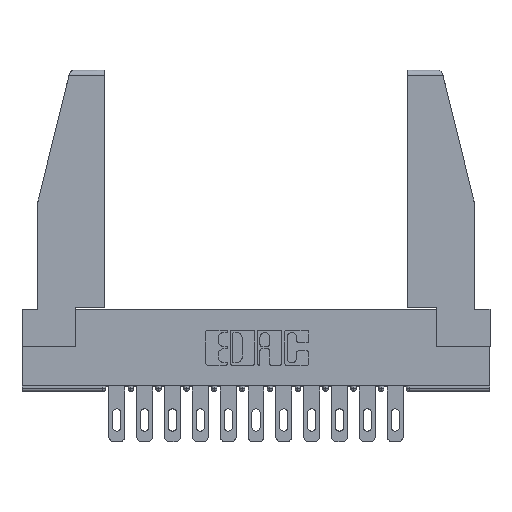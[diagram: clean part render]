
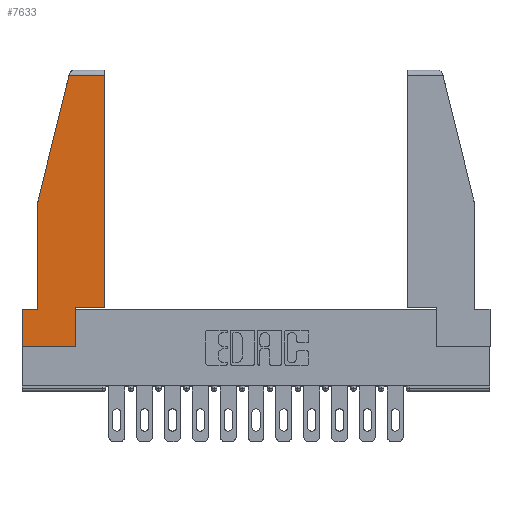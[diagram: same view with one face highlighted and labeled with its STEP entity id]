
A CAD part, top view. The second image highlights one B-rep face of the part: STEP entity #7633.
In plain terms, the highlighted planar face has unit normal (0, 0, 1).
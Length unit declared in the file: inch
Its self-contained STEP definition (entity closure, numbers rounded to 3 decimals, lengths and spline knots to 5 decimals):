
#5 = CARTESIAN_POINT ( 'NONE',  ( 0.086, 0.8, 0. ) ) ;
#120 = CARTESIAN_POINT ( 'NONE',  ( 0., 0., 0. ) ) ;
#125 = VECTOR ( 'NONE', #3399, 39.37008 ) ;
#659 = VERTEX_POINT ( 'NONE', #16445 ) ;
#862 = DIRECTION ( 'NONE',  ( -1., 0., 0. ) ) ;
#889 = ORIENTED_EDGE ( 'NONE', *, *, #14998, .T. ) ;
#1117 = LINE ( 'NONE', #10937, #11453 ) ;
#1218 = CARTESIAN_POINT ( 'NONE',  ( 0., 0.21, 0. ) ) ;
#1313 = VECTOR ( 'NONE', #11374, 39.37008 ) ;
#1883 = EDGE_CURVE ( 'NONE', #5076, #17336, #9200, .T. ) ;
#2120 = LINE ( 'NONE', #8491, #6727 ) ;
#2678 = LINE ( 'NONE', #7862, #3133 ) ;
#2853 = LINE ( 'NONE', #5, #1313 ) ;
#2906 = DIRECTION ( 'NONE',  ( 1., 0., 0. ) ) ;
#2935 = ORIENTED_EDGE ( 'NONE', *, *, #14769, .T. ) ;
#2953 = ORIENTED_EDGE ( 'NONE', *, *, #5495, .T. ) ;
#3133 = VECTOR ( 'NONE', #862, 39.37008 ) ;
#3399 = DIRECTION ( 'NONE',  ( -0.239, -0.971, 0. ) ) ;
#4115 = VERTEX_POINT ( 'NONE', #8168 ) ;
#4915 = DIRECTION ( 'NONE',  ( 0., 1., 0. ) ) ;
#5076 = VERTEX_POINT ( 'NONE', #9344 ) ;
#5495 = EDGE_CURVE ( 'NONE', #17336, #659, #12413, .T. ) ;
#5651 = EDGE_CURVE ( 'NONE', #8223, #5076, #15651, .T. ) ;
#5708 = PLANE ( 'NONE',  #13709 ) ;
#5934 = CARTESIAN_POINT ( 'NONE',  ( 0.461, 0.223, 0. ) ) ;
#6173 = VERTEX_POINT ( 'NONE', #17697 ) ;
#6325 = CARTESIAN_POINT ( 'NONE',  ( 0.297, 0., 0. ) ) ;
#6475 = EDGE_LOOP ( 'NONE', ( #2953, #10082, #889, #10872, #17646, #7102, #2935, #10143, #6641 ) ) ;
#6641 = ORIENTED_EDGE ( 'NONE', *, *, #1883, .T. ) ;
#6727 = VECTOR ( 'NONE', #2906, 39.37008 ) ;
#7102 = ORIENTED_EDGE ( 'NONE', *, *, #12108, .T. ) ;
#7633 = ADVANCED_FACE ( 'NONE', ( #17396 ), #5708, .T. ) ;
#7862 = CARTESIAN_POINT ( 'NONE',  ( 0., 1.52, 0. ) ) ;
#8168 = CARTESIAN_POINT ( 'NONE',  ( 0., 0., 0. ) ) ;
#8223 = VERTEX_POINT ( 'NONE', #6325 ) ;
#8384 = DIRECTION ( 'NONE',  ( 1., 0., 0. ) ) ;
#8491 = CARTESIAN_POINT ( 'NONE',  ( 0., 0., 0. ) ) ;
#8547 = CARTESIAN_POINT ( 'NONE',  ( 0.086, 0.8, 0. ) ) ;
#8592 = DIRECTION ( 'NONE',  ( 0., 0., 1. ) ) ;
#8653 = DIRECTION ( 'NONE',  ( 1., 0., 0. ) ) ;
#9200 = LINE ( 'NONE', #16771, #12053 ) ;
#9232 = VERTEX_POINT ( 'NONE', #18126 ) ;
#9284 = VERTEX_POINT ( 'NONE', #9942 ) ;
#9344 = CARTESIAN_POINT ( 'NONE',  ( 0.297, 0.223, 0. ) ) ;
#9459 = DIRECTION ( 'NONE',  ( 0., -1., 0. ) ) ;
#9942 = CARTESIAN_POINT ( 'NONE',  ( 0.2636, 1.52, 0. ) ) ;
#10082 = ORIENTED_EDGE ( 'NONE', *, *, #17520, .T. ) ;
#10143 = ORIENTED_EDGE ( 'NONE', *, *, #5651, .T. ) ;
#10469 = LINE ( 'NONE', #11800, #125 ) ;
#10872 = ORIENTED_EDGE ( 'NONE', *, *, #12628, .T. ) ;
#10879 = DIRECTION ( 'NONE',  ( -1., 0., 0. ) ) ;
#10937 = CARTESIAN_POINT ( 'NONE',  ( 0., 0.21, 0. ) ) ;
#11321 = VECTOR ( 'NONE', #4915, 39.37008 ) ;
#11374 = DIRECTION ( 'NONE',  ( 0., -1., 0. ) ) ;
#11453 = VECTOR ( 'NONE', #9459, 39.37008 ) ;
#11800 = CARTESIAN_POINT ( 'NONE',  ( 0.271, 1.55, 0. ) ) ;
#12053 = VECTOR ( 'NONE', #8384, 39.37008 ) ;
#12108 = EDGE_CURVE ( 'NONE', #6173, #4115, #1117, .T. ) ;
#12193 = EDGE_CURVE ( 'NONE', #9232, #6173, #13627, .T. ) ;
#12413 = LINE ( 'NONE', #13131, #15005 ) ;
#12628 = EDGE_CURVE ( 'NONE', #15964, #9232, #2853, .T. ) ;
#13131 = CARTESIAN_POINT ( 'NONE',  ( 0.461, 0.223, 0. ) ) ;
#13188 = DIRECTION ( 'NONE',  ( 0., 1., 0. ) ) ;
#13627 = LINE ( 'NONE', #1218, #14492 ) ;
#13709 = AXIS2_PLACEMENT_3D ( 'NONE', #120, #8592, #8653 ) ;
#14492 = VECTOR ( 'NONE', #10879, 39.37008 ) ;
#14681 = CARTESIAN_POINT ( 'NONE',  ( 0.297, 0., 0. ) ) ;
#14769 = EDGE_CURVE ( 'NONE', #4115, #8223, #2120, .T. ) ;
#14998 = EDGE_CURVE ( 'NONE', #9284, #15964, #10469, .T. ) ;
#15005 = VECTOR ( 'NONE', #13188, 39.37008 ) ;
#15651 = LINE ( 'NONE', #14681, #11321 ) ;
#15964 = VERTEX_POINT ( 'NONE', #8547 ) ;
#16445 = CARTESIAN_POINT ( 'NONE',  ( 0.461, 1.52, 0. ) ) ;
#16771 = CARTESIAN_POINT ( 'NONE',  ( 0.297, 0.223, 0. ) ) ;
#17336 = VERTEX_POINT ( 'NONE', #5934 ) ;
#17396 = FACE_OUTER_BOUND ( 'NONE', #6475, .T. ) ;
#17520 = EDGE_CURVE ( 'NONE', #659, #9284, #2678, .T. ) ;
#17646 = ORIENTED_EDGE ( 'NONE', *, *, #12193, .T. ) ;
#17697 = CARTESIAN_POINT ( 'NONE',  ( 0., 0.21, 0. ) ) ;
#18126 = CARTESIAN_POINT ( 'NONE',  ( 0.086, 0.21, 0. ) ) ;
